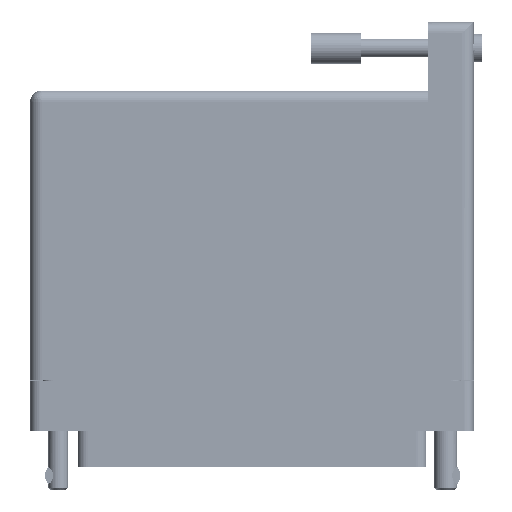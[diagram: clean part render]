
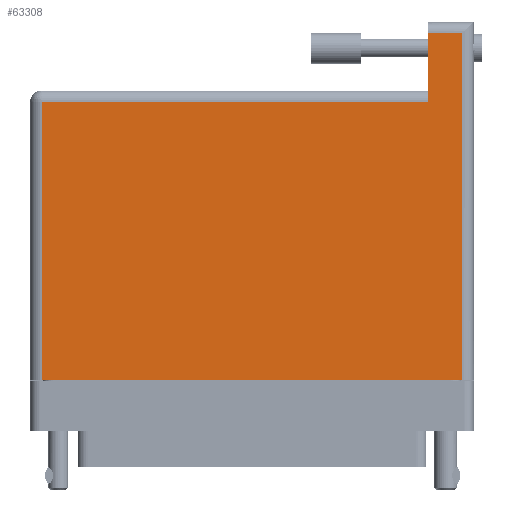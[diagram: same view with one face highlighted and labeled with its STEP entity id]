
A CAD part, front view. The second image highlights one B-rep face of the part: STEP entity #63308.
In plain terms, the highlighted face is planar.
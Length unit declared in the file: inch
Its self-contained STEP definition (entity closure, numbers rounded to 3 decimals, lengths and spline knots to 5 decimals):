
#599 = ORIENTED_EDGE ( 'NONE', *, *, #2202, .T. ) ;
#1023 = ORIENTED_EDGE ( 'NONE', *, *, #9876, .T. ) ;
#2202 = EDGE_CURVE ( 'NONE', #8462, #35188, #8397, .T. ) ;
#2362 = VECTOR ( 'NONE', #47924, 39.37008 ) ;
#3632 = CARTESIAN_POINT ( 'NONE',  ( -1.359, 1.675, 0.617 ) ) ;
#8397 = LINE ( 'NONE', #33554, #49891 ) ;
#8462 = VERTEX_POINT ( 'NONE', #53301 ) ;
#8983 = DIRECTION ( 'NONE',  ( 0., 0., -1. ) ) ;
#9876 = EDGE_CURVE ( 'NONE', #22389, #34516, #63636, .T. ) ;
#11632 = ORIENTED_EDGE ( 'NONE', *, *, #50330, .T. ) ;
#14574 = VECTOR ( 'NONE', #19084, 39.37008 ) ;
#14584 = EDGE_CURVE ( 'NONE', #54654, #82731, #79240, .T. ) ;
#14843 = LINE ( 'NONE', #71010, #74417 ) ;
#16487 = LINE ( 'NONE', #62706, #54840 ) ;
#19084 = DIRECTION ( 'NONE',  ( 0., 1., 0. ) ) ;
#19337 = DIRECTION ( 'NONE',  ( 1., 0., 0. ) ) ;
#21157 = VECTOR ( 'NONE', #36400, 39.37008 ) ;
#22389 = VERTEX_POINT ( 'NONE', #34451 ) ;
#25373 = EDGE_CURVE ( 'NONE', #82731, #8462, #33783, .T. ) ;
#28462 = CARTESIAN_POINT ( 'NONE',  ( -1.359, 2.025, 0.617 ) ) ;
#29894 = CARTESIAN_POINT ( 'NONE',  ( -1.289, -0.1, 0.617 ) ) ;
#30480 = ORIENTED_EDGE ( 'NONE', *, *, #35822, .T. ) ;
#30748 = ORIENTED_EDGE ( 'NONE', *, *, #25373, .T. ) ;
#33554 = CARTESIAN_POINT ( 'NONE',  ( 1.079, 2.095, 0.617 ) ) ;
#33783 = LINE ( 'NONE', #28462, #2362 ) ;
#34097 = DIRECTION ( 'NONE',  ( 0., -1., 0. ) ) ;
#34451 = CARTESIAN_POINT ( 'NONE',  ( -1.289, 1.605, 0.617 ) ) ;
#34516 = VERTEX_POINT ( 'NONE', #66216 ) ;
#35188 = VERTEX_POINT ( 'NONE', #36807 ) ;
#35822 = EDGE_CURVE ( 'NONE', #34516, #54654, #14843, .T. ) ;
#36400 = DIRECTION ( 'NONE',  ( 0., -1., 0. ) ) ;
#36807 = CARTESIAN_POINT ( 'NONE',  ( 1.079, 1.605, 0.617 ) ) ;
#42698 = DIRECTION ( 'NONE',  ( -1., 0., 0. ) ) ;
#44988 = EDGE_LOOP ( 'NONE', ( #11632, #1023, #30480, #49016, #30748, #599 ) ) ;
#47924 = DIRECTION ( 'NONE',  ( -1., 0., 0. ) ) ;
#49016 = ORIENTED_EDGE ( 'NONE', *, *, #14584, .T. ) ;
#49891 = VECTOR ( 'NONE', #34097, 39.37008 ) ;
#50330 = EDGE_CURVE ( 'NONE', #35188, #22389, #16487, .T. ) ;
#51800 = AXIS2_PLACEMENT_3D ( 'NONE', #3632, #8983, #61885 ) ;
#52024 = CARTESIAN_POINT ( 'NONE',  ( 1.289, 2.095, 0.617 ) ) ;
#53301 = CARTESIAN_POINT ( 'NONE',  ( 1.079, 2.025, 0.617 ) ) ;
#54654 = VERTEX_POINT ( 'NONE', #58628 ) ;
#54840 = VECTOR ( 'NONE', #42698, 39.37008 ) ;
#58186 = FACE_OUTER_BOUND ( 'NONE', #44988, .T. ) ;
#58628 = CARTESIAN_POINT ( 'NONE',  ( 1.289, -0.1, 0.617 ) ) ;
#61885 = DIRECTION ( 'NONE',  ( -1., 0., 0. ) ) ;
#62706 = CARTESIAN_POINT ( 'NONE',  ( -1.359, 1.605, 0.617 ) ) ;
#63308 = ADVANCED_FACE ( 'NONE', ( #58186 ), #74579, .F. ) ;
#63636 = LINE ( 'NONE', #29894, #21157 ) ;
#66216 = CARTESIAN_POINT ( 'NONE',  ( -1.289, -0.1, 0.617 ) ) ;
#71010 = CARTESIAN_POINT ( 'NONE',  ( -1.359, -0.1, 0.617 ) ) ;
#74417 = VECTOR ( 'NONE', #19337, 39.37008 ) ;
#74579 = PLANE ( 'NONE',  #51800 ) ;
#79240 = LINE ( 'NONE', #52024, #14574 ) ;
#81656 = CARTESIAN_POINT ( 'NONE',  ( 1.289, 2.025, 0.617 ) ) ;
#82731 = VERTEX_POINT ( 'NONE', #81656 ) ;
